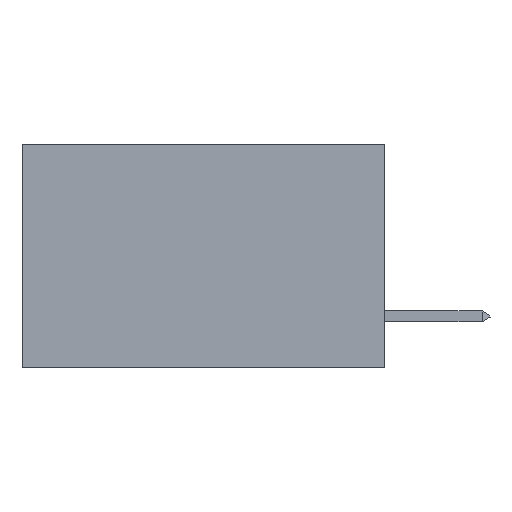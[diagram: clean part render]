
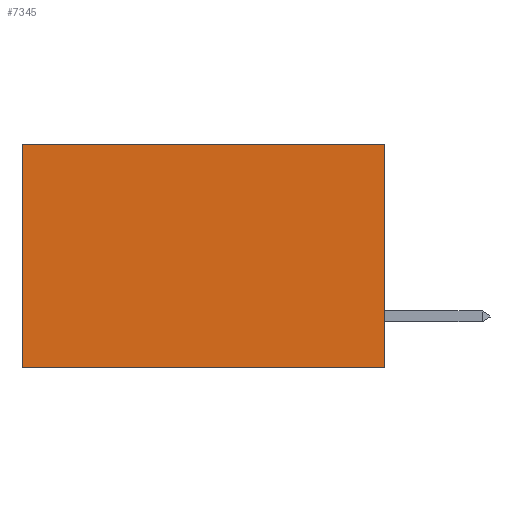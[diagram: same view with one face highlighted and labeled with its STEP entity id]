
A CAD part, left-side view. The second image highlights one B-rep face of the part: STEP entity #7345.
In plain terms, the highlighted planar face has unit normal (-1, 0, 0).
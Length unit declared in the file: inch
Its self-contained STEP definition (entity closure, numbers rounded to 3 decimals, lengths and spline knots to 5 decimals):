
#30 = DIRECTION ( 'NONE',  ( 0., 0., -1. ) ) ;
#1494 = CARTESIAN_POINT ( 'NONE',  ( 0.2875, 0., 0. ) ) ;
#1760 = DIRECTION ( 'NONE',  ( 0., 0., -1. ) ) ;
#2058 = EDGE_CURVE ( 'NONE', #6927, #6186, #7055, .T. ) ;
#2603 = DIRECTION ( 'NONE',  ( 0., 1., 0. ) ) ;
#2918 = DIRECTION ( 'NONE',  ( 0., 0., -1. ) ) ;
#2982 = EDGE_CURVE ( 'NONE', #6927, #6473, #6908, .T. ) ;
#3228 = ORIENTED_EDGE ( 'NONE', *, *, #2982, .F. ) ;
#3401 = CARTESIAN_POINT ( 'NONE',  ( 0.2875, 0., 0. ) ) ;
#3480 = EDGE_LOOP ( 'NONE', ( #8516, #5758, #3228, #6227 ) ) ;
#3531 = CARTESIAN_POINT ( 'NONE',  ( 0.2875, 0., -0.37 ) ) ;
#4428 = CARTESIAN_POINT ( 'NONE',  ( 0.2875, 0., 0. ) ) ;
#4446 = CARTESIAN_POINT ( 'NONE',  ( 0.2875, 0., 0. ) ) ;
#4578 = AXIS2_PLACEMENT_3D ( 'NONE', #1494, #7764, #30 ) ;
#4589 = CARTESIAN_POINT ( 'NONE',  ( 0.2875, 0.6, 0. ) ) ;
#4707 = FACE_OUTER_BOUND ( 'NONE', #3480, .T. ) ;
#4879 = PLANE ( 'NONE',  #4578 ) ;
#5590 = VECTOR ( 'NONE', #2918, 39.37008 ) ;
#5758 = ORIENTED_EDGE ( 'NONE', *, *, #7284, .F. ) ;
#6101 = CARTESIAN_POINT ( 'NONE',  ( 0.2875, 0.6, 0. ) ) ;
#6110 = CARTESIAN_POINT ( 'NONE',  ( 0.2875, 0.6, -0.37 ) ) ;
#6186 = VERTEX_POINT ( 'NONE', #6101 ) ;
#6227 = ORIENTED_EDGE ( 'NONE', *, *, #2058, .T. ) ;
#6473 = VERTEX_POINT ( 'NONE', #3531 ) ;
#6601 = EDGE_CURVE ( 'NONE', #6186, #7697, #8661, .T. ) ;
#6864 = CARTESIAN_POINT ( 'NONE',  ( 0.2875, 0., -0.37 ) ) ;
#6908 = LINE ( 'NONE', #4446, #5590 ) ;
#6927 = VERTEX_POINT ( 'NONE', #4428 ) ;
#7055 = LINE ( 'NONE', #3401, #7614 ) ;
#7284 = EDGE_CURVE ( 'NONE', #6473, #7697, #8075, .T. ) ;
#7286 = VECTOR ( 'NONE', #2603, 39.37008 ) ;
#7345 = ADVANCED_FACE ( 'NONE', ( #4707 ), #4879, .F. ) ;
#7614 = VECTOR ( 'NONE', #8194, 39.37008 ) ;
#7697 = VERTEX_POINT ( 'NONE', #6110 ) ;
#7764 = DIRECTION ( 'NONE',  ( 1., 0., 0. ) ) ;
#8075 = LINE ( 'NONE', #6864, #7286 ) ;
#8194 = DIRECTION ( 'NONE',  ( 0., 1., 0. ) ) ;
#8427 = VECTOR ( 'NONE', #1760, 39.37008 ) ;
#8516 = ORIENTED_EDGE ( 'NONE', *, *, #6601, .T. ) ;
#8661 = LINE ( 'NONE', #4589, #8427 ) ;
